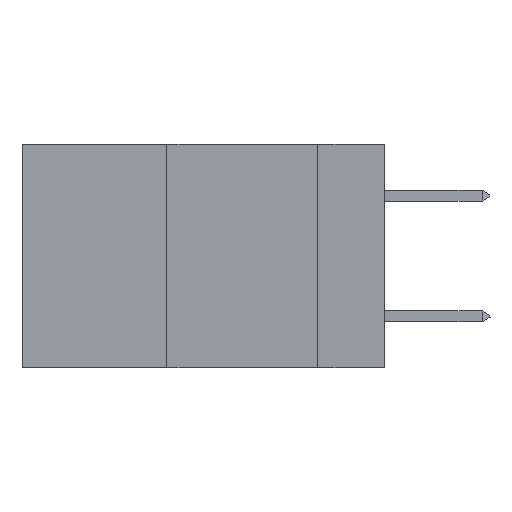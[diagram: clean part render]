
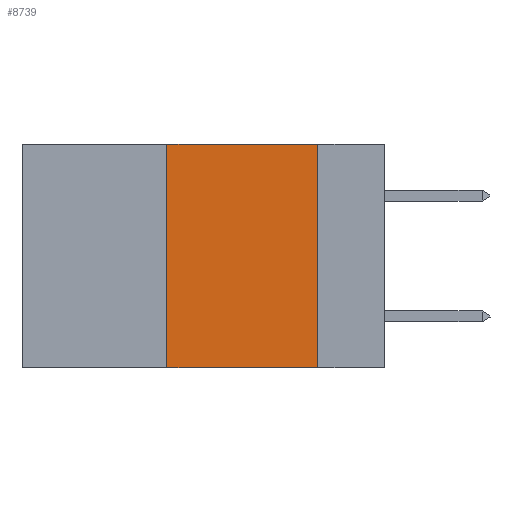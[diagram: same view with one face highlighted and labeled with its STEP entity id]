
A CAD part, left-side view. The second image highlights one B-rep face of the part: STEP entity #8739.
In plain terms, the highlighted planar face has unit normal (-1, 0, 0).
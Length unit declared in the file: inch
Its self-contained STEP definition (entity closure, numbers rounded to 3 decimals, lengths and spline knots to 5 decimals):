
#100 = FACE_OUTER_BOUND ( 'NONE', #5642, .T. ) ;
#705 = ORIENTED_EDGE ( 'NONE', *, *, #7931, .F. ) ;
#1981 = LINE ( 'NONE', #14880, #6491 ) ;
#1984 = LINE ( 'NONE', #6783, #3378 ) ;
#2244 = CARTESIAN_POINT ( 'NONE',  ( 0., 0.11, 0. ) ) ;
#3019 = LINE ( 'NONE', #13569, #13558 ) ;
#3378 = VECTOR ( 'NONE', #3971, 39.37008 ) ;
#3432 = ORIENTED_EDGE ( 'NONE', *, *, #3856, .F. ) ;
#3552 = ORIENTED_EDGE ( 'NONE', *, *, #14043, .F. ) ;
#3799 = VECTOR ( 'NONE', #7609, 39.37008 ) ;
#3856 = EDGE_CURVE ( 'NONE', #7075, #12143, #1984, .T. ) ;
#3965 = VERTEX_POINT ( 'NONE', #2244 ) ;
#3971 = DIRECTION ( 'NONE',  ( 0., 0., 1. ) ) ;
#4531 = DIRECTION ( 'NONE',  ( 1., 0., 0. ) ) ;
#5517 = CARTESIAN_POINT ( 'NONE',  ( 0., 0.36, -0.37 ) ) ;
#5633 = DIRECTION ( 'NONE',  ( 0., 0., -1. ) ) ;
#5642 = EDGE_LOOP ( 'NONE', ( #705, #3552, #3432, #8323 ) ) ;
#5795 = CARTESIAN_POINT ( 'NONE',  ( 0., 0.6, 0. ) ) ;
#6304 = CARTESIAN_POINT ( 'NONE',  ( 0., 0.36, 0. ) ) ;
#6491 = VECTOR ( 'NONE', #13653, 39.37008 ) ;
#6783 = CARTESIAN_POINT ( 'NONE',  ( 0., 0.36, 0. ) ) ;
#7075 = VERTEX_POINT ( 'NONE', #5517 ) ;
#7259 = EDGE_CURVE ( 'NONE', #7075, #13010, #1981, .T. ) ;
#7609 = DIRECTION ( 'NONE',  ( 0., -1., 0. ) ) ;
#7931 = EDGE_CURVE ( 'NONE', #3965, #13010, #3019, .T. ) ;
#7960 = AXIS2_PLACEMENT_3D ( 'NONE', #5795, #4531, #5633 ) ;
#8323 = ORIENTED_EDGE ( 'NONE', *, *, #7259, .T. ) ;
#8739 = ADVANCED_FACE ( 'NONE', ( #100 ), #10272, .F. ) ;
#10272 = PLANE ( 'NONE',  #7960 ) ;
#11093 = CARTESIAN_POINT ( 'NONE',  ( 0., 0.6, 0. ) ) ;
#12143 = VERTEX_POINT ( 'NONE', #6304 ) ;
#12330 = DIRECTION ( 'NONE',  ( 0., 0., -1. ) ) ;
#13010 = VERTEX_POINT ( 'NONE', #13638 ) ;
#13558 = VECTOR ( 'NONE', #12330, 39.37008 ) ;
#13569 = CARTESIAN_POINT ( 'NONE',  ( 0., 0.11, 0. ) ) ;
#13638 = CARTESIAN_POINT ( 'NONE',  ( 0., 0.11, -0.37 ) ) ;
#13653 = DIRECTION ( 'NONE',  ( 0., -1., 0. ) ) ;
#14043 = EDGE_CURVE ( 'NONE', #12143, #3965, #14372, .T. ) ;
#14372 = LINE ( 'NONE', #11093, #3799 ) ;
#14880 = CARTESIAN_POINT ( 'NONE',  ( 0., 0.6, -0.37 ) ) ;
